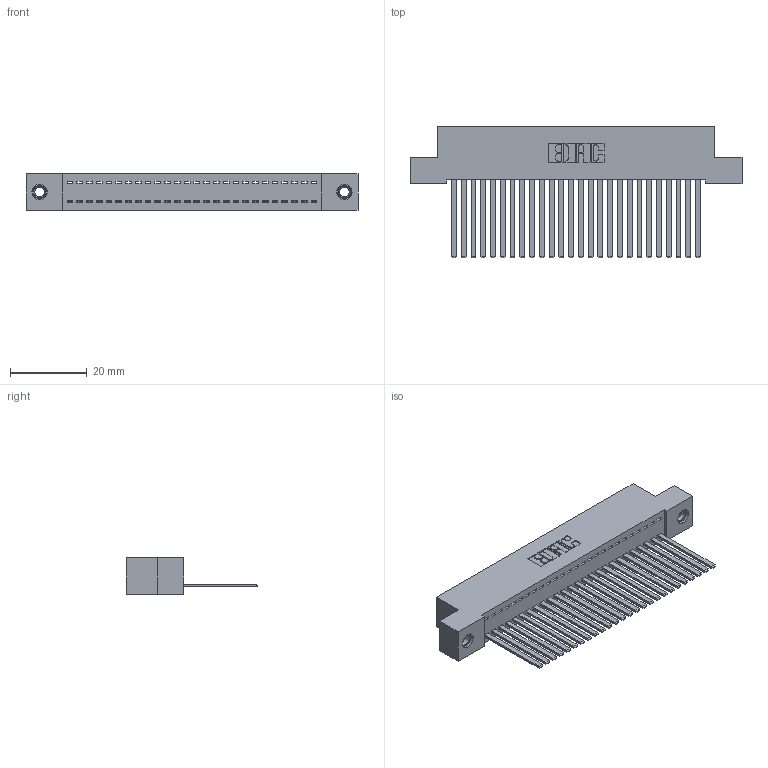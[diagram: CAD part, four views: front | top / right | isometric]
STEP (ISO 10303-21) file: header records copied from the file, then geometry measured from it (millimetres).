
FILE_DESCRIPTION (( 'STEP AP203' ), '1' );
FILE_NAME ('342-026-544-107.STEP', '2018-08-11T04:51:04', ( '' ), ( '' ), 'SwSTEP 2.0', 'SolidWorks 2016', '' );
FILE_SCHEMA (( 'CONFIG_CONTROL_DESIGN' ));
Length unit declared in the file: inch
Products named in the file (4): 342-026-544-107; 342 Part_TI; 345-292-001_345-293-144; 345-250-001_345-250-005-103
Assembly tree (29 placements, depth 2):
  342-026-544-107
    342 Part_TI
    345-292-001_345-293-144  x26
    345-250-001_345-250-005-103  x2
Bounding box: 86.36 x 34.3 x 9.4 mm (x, y, z)
Volume: 7801.5 mm3; surface area: 12046.7 mm2
Topology: 29 solids, 29 shells, 1522 faces, 4543 edges, 2986 vertices
Faces by surface type: plane 1086, cylinder 420, cone 12, torus 4
Entity records: 18834 total; most frequent: CARTESIAN_POINT 3231, ORIENTED_EDGE 3186, DIRECTION 2787, EDGE_CURVE 1593, LINE 1449, VECTOR 1449, VERTEX_POINT 1056, AXIS2_PLACEMENT_3D 669
